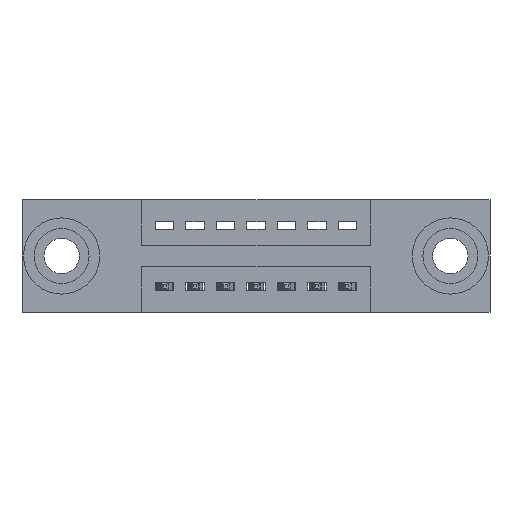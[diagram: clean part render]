
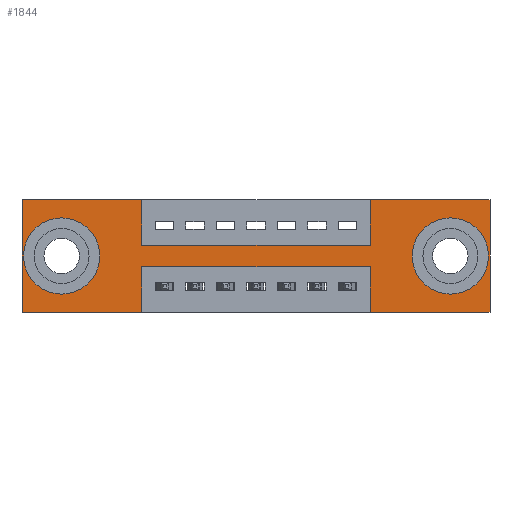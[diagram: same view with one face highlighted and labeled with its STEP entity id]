
A CAD part, front view. The second image highlights one B-rep face of the part: STEP entity #1844.
In plain terms, the highlighted planar face has unit normal (0, -1, 0).
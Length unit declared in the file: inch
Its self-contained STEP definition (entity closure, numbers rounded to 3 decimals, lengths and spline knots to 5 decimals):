
#23 = DIRECTION ( 'NONE',  ( 0., 0., 1. ) ) ;
#153 = VECTOR ( 'NONE', #9352, 39.37008 ) ;
#332 = VECTOR ( 'NONE', #6789, 39.37008 ) ;
#411 = DIRECTION ( 'NONE',  ( 1., 0., 0. ) ) ;
#570 = EDGE_LOOP ( 'NONE', ( #9207, #9330, #4125, #6419, #8604, #9467, #3895, #3967, #7163, #4633, #4425, #5440 ) ) ;
#614 = CARTESIAN_POINT ( 'NONE',  ( 0., 0., -0.37 ) ) ;
#652 = VERTEX_POINT ( 'NONE', #10372 ) ;
#764 = CARTESIAN_POINT ( 'NONE',  ( 1.405, 0., -0.185 ) ) ;
#881 = VECTOR ( 'NONE', #5490, 39.37008 ) ;
#887 = AXIS2_PLACEMENT_3D ( 'NONE', #614, #1394, #2327 ) ;
#906 = VERTEX_POINT ( 'NONE', #5067 ) ;
#980 = LINE ( 'NONE', #5438, #332 ) ;
#989 = VECTOR ( 'NONE', #23, 39.37008 ) ;
#1017 = CARTESIAN_POINT ( 'NONE',  ( 1.1425, 0., -0.37 ) ) ;
#1118 = FACE_OUTER_BOUND ( 'NONE', #570, .T. ) ;
#1359 = CARTESIAN_POINT ( 'NONE',  ( 1.1425, 0., -0.37 ) ) ;
#1394 = DIRECTION ( 'NONE',  ( 0., -1., 0. ) ) ;
#1405 = CARTESIAN_POINT ( 'NONE',  ( 0.3925, 0., 0. ) ) ;
#1462 = CARTESIAN_POINT ( 'NONE',  ( 0.3925, 0., -0.22 ) ) ;
#1464 = CARTESIAN_POINT ( 'NONE',  ( 0., 0., 0. ) ) ;
#1491 = DIRECTION ( 'NONE',  ( 0., 0., -1. ) ) ;
#1506 = DIRECTION ( 'NONE',  ( -1., 0., 0. ) ) ;
#1508 = CARTESIAN_POINT ( 'NONE',  ( 0.13, 0., -0.263 ) ) ;
#1542 = DIRECTION ( 'NONE',  ( 0., 0., -1. ) ) ;
#1618 = DIRECTION ( 'NONE',  ( 1., 0., 0. ) ) ;
#1669 = CARTESIAN_POINT ( 'NONE',  ( 0.13, 0., -0.185 ) ) ;
#1770 = VECTOR ( 'NONE', #10435, 39.37008 ) ;
#1844 = ADVANCED_FACE ( 'NONE', ( #8462, #6240, #1118 ), #6376, .T. ) ;
#1858 = EDGE_CURVE ( 'NONE', #3834, #2219, #7419, .T. ) ;
#2093 = VECTOR ( 'NONE', #7079, 39.37008 ) ;
#2132 = VERTEX_POINT ( 'NONE', #9298 ) ;
#2182 = DIRECTION ( 'NONE',  ( 0., 0., 1. ) ) ;
#2219 = VERTEX_POINT ( 'NONE', #3632 ) ;
#2316 = LINE ( 'NONE', #3597, #153 ) ;
#2327 = DIRECTION ( 'NONE',  ( 0., 0., -1. ) ) ;
#2473 = DIRECTION ( 'NONE',  ( 0., 0., 1. ) ) ;
#2500 = EDGE_CURVE ( 'NONE', #9389, #7017, #10122, .T. ) ;
#2540 = CARTESIAN_POINT ( 'NONE',  ( 0.3925, 0., -0.37 ) ) ;
#2586 = CARTESIAN_POINT ( 'NONE',  ( 0.3925, 0., 0. ) ) ;
#2667 = VERTEX_POINT ( 'NONE', #6736 ) ;
#2817 = CARTESIAN_POINT ( 'NONE',  ( 1.535, 0., 0. ) ) ;
#2827 = LINE ( 'NONE', #1462, #9517 ) ;
#2834 = CARTESIAN_POINT ( 'NONE',  ( 0., 0., 0. ) ) ;
#3067 = VERTEX_POINT ( 'NONE', #2586 ) ;
#3149 = LINE ( 'NONE', #8191, #989 ) ;
#3163 = EDGE_CURVE ( 'NONE', #7243, #3067, #7770, .T. ) ;
#3393 = EDGE_CURVE ( 'NONE', #4249, #4026, #3149, .T. ) ;
#3491 = EDGE_CURVE ( 'NONE', #9985, #9389, #980, .T. ) ;
#3597 = CARTESIAN_POINT ( 'NONE',  ( 1.535, 0., 0. ) ) ;
#3632 = CARTESIAN_POINT ( 'NONE',  ( 1.1425, 0., -0.22 ) ) ;
#3770 = LINE ( 'NONE', #6233, #6620 ) ;
#3834 = VERTEX_POINT ( 'NONE', #1017 ) ;
#3895 = ORIENTED_EDGE ( 'NONE', *, *, #3393, .F. ) ;
#3906 = DIRECTION ( 'NONE',  ( 0., 1., 0. ) ) ;
#3967 = ORIENTED_EDGE ( 'NONE', *, *, #6258, .F. ) ;
#4026 = VERTEX_POINT ( 'NONE', #6019 ) ;
#4125 = ORIENTED_EDGE ( 'NONE', *, *, #1858, .F. ) ;
#4227 = LINE ( 'NONE', #9794, #10531 ) ;
#4249 = VERTEX_POINT ( 'NONE', #9691 ) ;
#4303 = ORIENTED_EDGE ( 'NONE', *, *, #6133, .T. ) ;
#4390 = LINE ( 'NONE', #2834, #10309 ) ;
#4425 = ORIENTED_EDGE ( 'NONE', *, *, #7875, .F. ) ;
#4479 = EDGE_CURVE ( 'NONE', #4026, #6863, #4390, .T. ) ;
#4598 = EDGE_CURVE ( 'NONE', #3067, #2132, #6606, .T. ) ;
#4632 = AXIS2_PLACEMENT_3D ( 'NONE', #764, #7317, #1542 ) ;
#4633 = ORIENTED_EDGE ( 'NONE', *, *, #3163, .F. ) ;
#4662 = CARTESIAN_POINT ( 'NONE',  ( 0., 0., -0.37 ) ) ;
#4672 = VECTOR ( 'NONE', #2182, 39.37008 ) ;
#4712 = CARTESIAN_POINT ( 'NONE',  ( 0.3925, 0., -0.22 ) ) ;
#4742 = CIRCLE ( 'NONE', #4632, 0.078 ) ;
#4926 = DIRECTION ( 'NONE',  ( 0., 1., 0. ) ) ;
#5067 = CARTESIAN_POINT ( 'NONE',  ( 1.535, 0., -0.37 ) ) ;
#5438 = CARTESIAN_POINT ( 'NONE',  ( 0.3925, 0., -0.37 ) ) ;
#5440 = ORIENTED_EDGE ( 'NONE', *, *, #2500, .F. ) ;
#5444 = EDGE_CURVE ( 'NONE', #2219, #9985, #2827, .T. ) ;
#5490 = DIRECTION ( 'NONE',  ( -1., 0., 0. ) ) ;
#5539 = ORIENTED_EDGE ( 'NONE', *, *, #5561, .T. ) ;
#5561 = EDGE_CURVE ( 'NONE', #652, #2667, #4742, .T. ) ;
#5582 = AXIS2_PLACEMENT_3D ( 'NONE', #1669, #4926, #2473 ) ;
#5632 = CARTESIAN_POINT ( 'NONE',  ( 0., 0., -0.37 ) ) ;
#5766 = EDGE_LOOP ( 'NONE', ( #10303, #7536 ) ) ;
#5819 = EDGE_CURVE ( 'NONE', #6863, #906, #2316, .T. ) ;
#5901 = VERTEX_POINT ( 'NONE', #10282 ) ;
#6019 = CARTESIAN_POINT ( 'NONE',  ( 1.1425, 0., 0. ) ) ;
#6133 = EDGE_CURVE ( 'NONE', #2667, #652, #6412, .T. ) ;
#6233 = CARTESIAN_POINT ( 'NONE',  ( 0., 0., 0. ) ) ;
#6240 = FACE_BOUND ( 'NONE', #5766, .T. ) ;
#6258 = EDGE_CURVE ( 'NONE', #2132, #4249, #4227, .T. ) ;
#6373 = DIRECTION ( 'NONE',  ( 0., 0., 1. ) ) ;
#6376 = PLANE ( 'NONE',  #887 ) ;
#6412 = CIRCLE ( 'NONE', #6813, 0.078 ) ;
#6419 = ORIENTED_EDGE ( 'NONE', *, *, #7338, .F. ) ;
#6545 = VERTEX_POINT ( 'NONE', #1508 ) ;
#6606 = LINE ( 'NONE', #1405, #2093 ) ;
#6620 = VECTOR ( 'NONE', #6373, 39.37008 ) ;
#6694 = LINE ( 'NONE', #9610, #8380 ) ;
#6736 = CARTESIAN_POINT ( 'NONE',  ( 1.405, 0., -0.107 ) ) ;
#6789 = DIRECTION ( 'NONE',  ( 0., 0., -1. ) ) ;
#6813 = AXIS2_PLACEMENT_3D ( 'NONE', #7353, #8181, #1491 ) ;
#6863 = VERTEX_POINT ( 'NONE', #2817 ) ;
#7017 = VERTEX_POINT ( 'NONE', #4662 ) ;
#7027 = AXIS2_PLACEMENT_3D ( 'NONE', #8770, #3906, #7216 ) ;
#7079 = DIRECTION ( 'NONE',  ( 0., 0., -1. ) ) ;
#7149 = EDGE_LOOP ( 'NONE', ( #4303, #5539 ) ) ;
#7163 = ORIENTED_EDGE ( 'NONE', *, *, #4598, .F. ) ;
#7216 = DIRECTION ( 'NONE',  ( 0., 0., 1. ) ) ;
#7243 = VERTEX_POINT ( 'NONE', #9638 ) ;
#7317 = DIRECTION ( 'NONE',  ( 0., 1., 0. ) ) ;
#7338 = EDGE_CURVE ( 'NONE', #906, #3834, #6694, .T. ) ;
#7353 = CARTESIAN_POINT ( 'NONE',  ( 1.405, 0., -0.185 ) ) ;
#7419 = LINE ( 'NONE', #1359, #4672 ) ;
#7536 = ORIENTED_EDGE ( 'NONE', *, *, #8509, .T. ) ;
#7770 = LINE ( 'NONE', #1464, #1770 ) ;
#7875 = EDGE_CURVE ( 'NONE', #7017, #7243, #3770, .T. ) ;
#8181 = DIRECTION ( 'NONE',  ( 0., 1., 0. ) ) ;
#8191 = CARTESIAN_POINT ( 'NONE',  ( 1.1425, 0., 0. ) ) ;
#8380 = VECTOR ( 'NONE', #1506, 39.37008 ) ;
#8417 = CIRCLE ( 'NONE', #7027, 0.078 ) ;
#8462 = FACE_BOUND ( 'NONE', #7149, .T. ) ;
#8509 = EDGE_CURVE ( 'NONE', #6545, #5901, #8417, .T. ) ;
#8604 = ORIENTED_EDGE ( 'NONE', *, *, #5819, .F. ) ;
#8770 = CARTESIAN_POINT ( 'NONE',  ( 0.13, 0., -0.185 ) ) ;
#9207 = ORIENTED_EDGE ( 'NONE', *, *, #3491, .F. ) ;
#9298 = CARTESIAN_POINT ( 'NONE',  ( 0.3925, 0., -0.15 ) ) ;
#9330 = ORIENTED_EDGE ( 'NONE', *, *, #5444, .F. ) ;
#9352 = DIRECTION ( 'NONE',  ( 0., 0., -1. ) ) ;
#9389 = VERTEX_POINT ( 'NONE', #2540 ) ;
#9467 = ORIENTED_EDGE ( 'NONE', *, *, #4479, .F. ) ;
#9512 = CIRCLE ( 'NONE', #5582, 0.078 ) ;
#9517 = VECTOR ( 'NONE', #9607, 39.37008 ) ;
#9607 = DIRECTION ( 'NONE',  ( -1., 0., 0. ) ) ;
#9610 = CARTESIAN_POINT ( 'NONE',  ( 0., 0., -0.37 ) ) ;
#9638 = CARTESIAN_POINT ( 'NONE',  ( 0., 0., 0. ) ) ;
#9691 = CARTESIAN_POINT ( 'NONE',  ( 1.1425, 0., -0.15 ) ) ;
#9794 = CARTESIAN_POINT ( 'NONE',  ( 0.3925, 0., -0.15 ) ) ;
#9985 = VERTEX_POINT ( 'NONE', #4712 ) ;
#10096 = EDGE_CURVE ( 'NONE', #5901, #6545, #9512, .T. ) ;
#10122 = LINE ( 'NONE', #5632, #881 ) ;
#10282 = CARTESIAN_POINT ( 'NONE',  ( 0.13, 0., -0.107 ) ) ;
#10303 = ORIENTED_EDGE ( 'NONE', *, *, #10096, .T. ) ;
#10309 = VECTOR ( 'NONE', #411, 39.37008 ) ;
#10372 = CARTESIAN_POINT ( 'NONE',  ( 1.405, 0., -0.263 ) ) ;
#10435 = DIRECTION ( 'NONE',  ( 1., 0., 0. ) ) ;
#10531 = VECTOR ( 'NONE', #1618, 39.37008 ) ;
